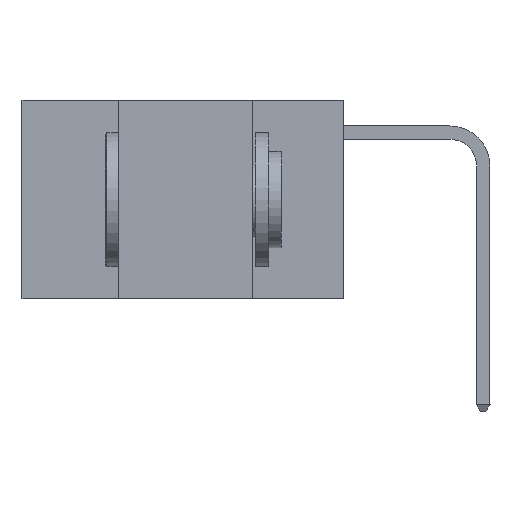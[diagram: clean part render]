
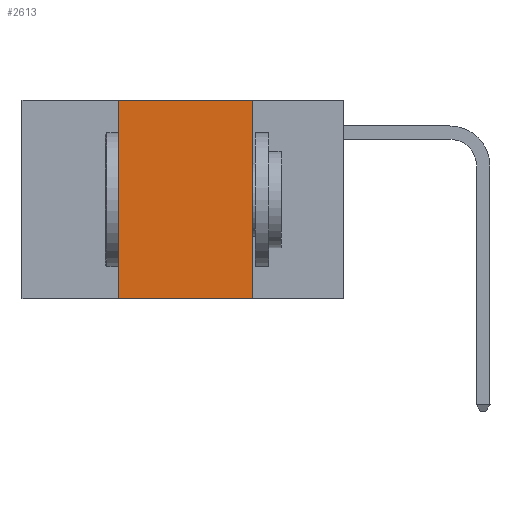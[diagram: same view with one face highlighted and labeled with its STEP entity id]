
A CAD part, left-side view. The second image highlights one B-rep face of the part: STEP entity #2613.
In plain terms, the highlighted planar face has unit normal (-1, 0, 0).
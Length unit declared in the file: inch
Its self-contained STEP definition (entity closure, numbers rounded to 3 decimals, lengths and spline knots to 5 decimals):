
#1035 = CARTESIAN_POINT ( 'NONE',  ( 0., 0.42, -0.37 ) ) ;
#1249 = DIRECTION ( 'NONE',  ( 0., 0., -1. ) ) ;
#1262 = DIRECTION ( 'NONE',  ( 1., 0., 0. ) ) ;
#1286 = PLANE ( 'NONE',  #1620 ) ;
#1323 = CARTESIAN_POINT ( 'NONE',  ( 0., 0.6, 0. ) ) ;
#1517 = FACE_OUTER_BOUND ( 'NONE', #4459, .T. ) ;
#1620 = AXIS2_PLACEMENT_3D ( 'NONE', #1323, #1262, #1249 ) ;
#1879 = ORIENTED_EDGE ( 'NONE', *, *, #9066, .F. ) ;
#1943 = VECTOR ( 'NONE', #9347, 39.37008 ) ;
#2033 = LINE ( 'NONE', #7106, #1943 ) ;
#2613 = ADVANCED_FACE ( 'NONE', ( #1517 ), #1286, .F. ) ;
#2828 = CARTESIAN_POINT ( 'NONE',  ( 0., 0.17, 0. ) ) ;
#2997 = CARTESIAN_POINT ( 'NONE',  ( 0., 0.6, 0. ) ) ;
#3093 = DIRECTION ( 'NONE',  ( 0., -1., 0. ) ) ;
#3552 = DIRECTION ( 'NONE',  ( 0., 0., -1. ) ) ;
#3674 = VECTOR ( 'NONE', #3552, 39.37008 ) ;
#3782 = LINE ( 'NONE', #2828, #3674 ) ;
#3910 = VECTOR ( 'NONE', #3093, 39.37008 ) ;
#4173 = VERTEX_POINT ( 'NONE', #6184 ) ;
#4196 = LINE ( 'NONE', #2997, #3910 ) ;
#4459 = EDGE_LOOP ( 'NONE', ( #8870, #9188, #1879, #5324 ) ) ;
#4473 = CARTESIAN_POINT ( 'NONE',  ( 0., 0.17, -0.37 ) ) ;
#4487 = VERTEX_POINT ( 'NONE', #5970 ) ;
#5174 = EDGE_CURVE ( 'NONE', #6371, #5815, #5846, .T. ) ;
#5324 = ORIENTED_EDGE ( 'NONE', *, *, #5174, .T. ) ;
#5810 = VECTOR ( 'NONE', #6125, 39.37008 ) ;
#5815 = VERTEX_POINT ( 'NONE', #4473 ) ;
#5839 = EDGE_CURVE ( 'NONE', #4487, #5815, #3782, .T. ) ;
#5846 = LINE ( 'NONE', #6118, #5810 ) ;
#5970 = CARTESIAN_POINT ( 'NONE',  ( 0., 0.17, 0. ) ) ;
#6118 = CARTESIAN_POINT ( 'NONE',  ( 0., 0.6, -0.37 ) ) ;
#6125 = DIRECTION ( 'NONE',  ( 0., -1., 0. ) ) ;
#6184 = CARTESIAN_POINT ( 'NONE',  ( 0., 0.42, 0. ) ) ;
#6371 = VERTEX_POINT ( 'NONE', #1035 ) ;
#7106 = CARTESIAN_POINT ( 'NONE',  ( 0., 0.42, 0. ) ) ;
#7498 = EDGE_CURVE ( 'NONE', #4173, #4487, #4196, .T. ) ;
#8870 = ORIENTED_EDGE ( 'NONE', *, *, #5839, .F. ) ;
#9066 = EDGE_CURVE ( 'NONE', #6371, #4173, #2033, .T. ) ;
#9188 = ORIENTED_EDGE ( 'NONE', *, *, #7498, .F. ) ;
#9347 = DIRECTION ( 'NONE',  ( 0., 0., 1. ) ) ;
